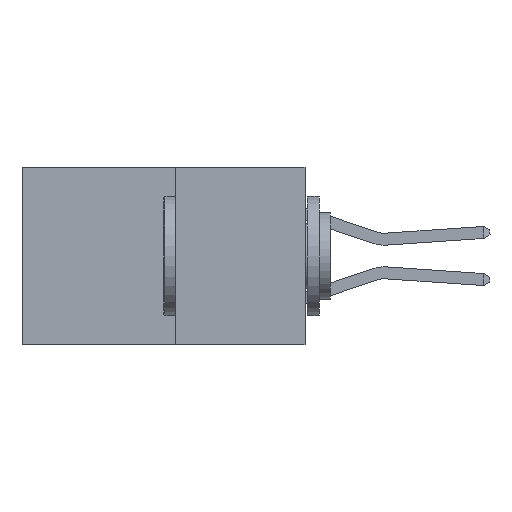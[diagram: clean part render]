
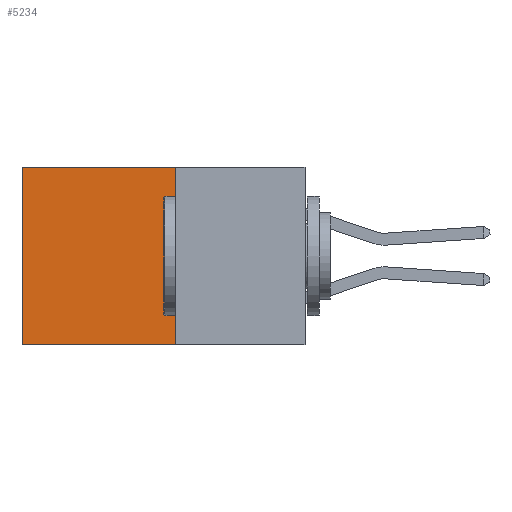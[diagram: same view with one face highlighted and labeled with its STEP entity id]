
A CAD part, left-side view. The second image highlights one B-rep face of the part: STEP entity #5234.
In plain terms, the highlighted planar face has unit normal (-1, 0, 0).
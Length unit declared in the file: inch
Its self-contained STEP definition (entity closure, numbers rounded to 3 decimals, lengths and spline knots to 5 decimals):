
#263 = VERTEX_POINT ( 'NONE', #20093 ) ;
#1334 = CARTESIAN_POINT ( 'NONE',  ( 0.277, 0.59, -0.37 ) ) ;
#3502 = EDGE_LOOP ( 'NONE', ( #22244, #17128, #15248, #12412 ) ) ;
#3626 = CARTESIAN_POINT ( 'NONE',  ( 0.277, 0.59, -0.37 ) ) ;
#3800 = VECTOR ( 'NONE', #3834, 39.37008 ) ;
#3834 = DIRECTION ( 'NONE',  ( 0., 0., -1. ) ) ;
#4721 = AXIS2_PLACEMENT_3D ( 'NONE', #7479, #7138, #7134 ) ;
#5234 = ADVANCED_FACE ( 'NONE', ( #16077 ), #7686, .F. ) ;
#5830 = LINE ( 'NONE', #25604, #23946 ) ;
#6107 = LINE ( 'NONE', #12395, #11907 ) ;
#6593 = VERTEX_POINT ( 'NONE', #8768 ) ;
#7134 = DIRECTION ( 'NONE',  ( 0., 0., -1. ) ) ;
#7138 = DIRECTION ( 'NONE',  ( 1., 0., 0. ) ) ;
#7446 = DIRECTION ( 'NONE',  ( 0., 0., -1. ) ) ;
#7479 = CARTESIAN_POINT ( 'NONE',  ( 0.277, 0.27, -0.37 ) ) ;
#7686 = PLANE ( 'NONE',  #4721 ) ;
#8375 = DIRECTION ( 'NONE',  ( 0., 1., 0. ) ) ;
#8523 = EDGE_CURVE ( 'NONE', #12635, #6593, #6107, .T. ) ;
#8768 = CARTESIAN_POINT ( 'NONE',  ( 0.277, 0.27, -0.37 ) ) ;
#11907 = VECTOR ( 'NONE', #7446, 39.37008 ) ;
#11959 = VECTOR ( 'NONE', #15864, 39.37008 ) ;
#12395 = CARTESIAN_POINT ( 'NONE',  ( 0.277, 0.27, -0.37 ) ) ;
#12412 = ORIENTED_EDGE ( 'NONE', *, *, #24395, .T. ) ;
#12635 = VERTEX_POINT ( 'NONE', #27727 ) ;
#13286 = EDGE_CURVE ( 'NONE', #6593, #29342, #5830, .T. ) ;
#15248 = ORIENTED_EDGE ( 'NONE', *, *, #8523, .F. ) ;
#15864 = DIRECTION ( 'NONE',  ( 0., 1., 0. ) ) ;
#16077 = FACE_OUTER_BOUND ( 'NONE', #3502, .T. ) ;
#17128 = ORIENTED_EDGE ( 'NONE', *, *, #13286, .F. ) ;
#17192 = EDGE_CURVE ( 'NONE', #263, #29342, #23503, .T. ) ;
#20093 = CARTESIAN_POINT ( 'NONE',  ( 0.277, 0.59, 0. ) ) ;
#22244 = ORIENTED_EDGE ( 'NONE', *, *, #17192, .T. ) ;
#23503 = LINE ( 'NONE', #1334, #3800 ) ;
#23946 = VECTOR ( 'NONE', #8375, 39.37008 ) ;
#24395 = EDGE_CURVE ( 'NONE', #12635, #263, #30652, .T. ) ;
#25604 = CARTESIAN_POINT ( 'NONE',  ( 0.277, 0.27, -0.37 ) ) ;
#27727 = CARTESIAN_POINT ( 'NONE',  ( 0.277, 0.27, 0. ) ) ;
#29342 = VERTEX_POINT ( 'NONE', #3626 ) ;
#30412 = CARTESIAN_POINT ( 'NONE',  ( 0.277, 0.27, 0. ) ) ;
#30652 = LINE ( 'NONE', #30412, #11959 ) ;
